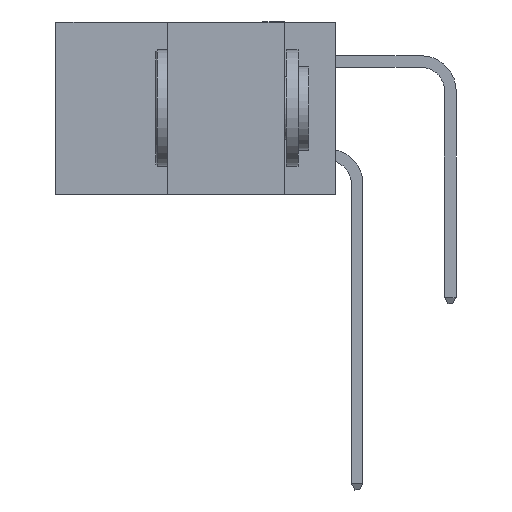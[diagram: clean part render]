
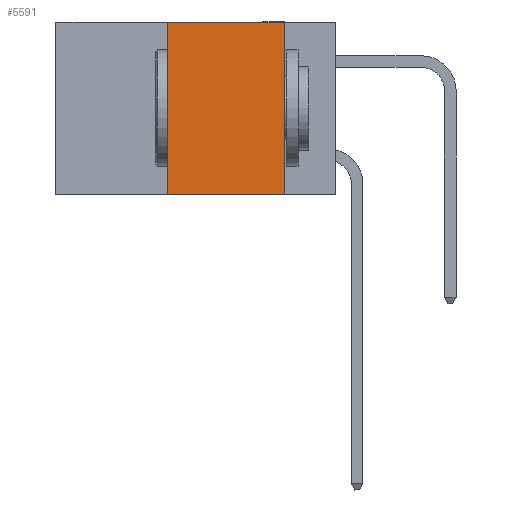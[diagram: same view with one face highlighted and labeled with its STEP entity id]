
A CAD part, left-side view. The second image highlights one B-rep face of the part: STEP entity #5591.
In plain terms, the highlighted planar face has unit normal (-1, 0, 0).
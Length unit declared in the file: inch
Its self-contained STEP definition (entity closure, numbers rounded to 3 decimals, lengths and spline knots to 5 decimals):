
#1608 = VECTOR ( 'NONE', #17284, 39.37008 ) ;
#1624 = LINE ( 'NONE', #6022, #5267 ) ;
#1703 = EDGE_LOOP ( 'NONE', ( #5693, #5803, #6019, #6111 ) ) ;
#1798 = CARTESIAN_POINT ( 'NONE',  ( 0., 0.6, 0. ) ) ;
#2608 = VECTOR ( 'NONE', #3394, 39.37008 ) ;
#2802 = VERTEX_POINT ( 'NONE', #12249 ) ;
#3334 = PLANE ( 'NONE',  #11237 ) ;
#3394 = DIRECTION ( 'NONE',  ( 0., -1., 0. ) ) ;
#5258 = VERTEX_POINT ( 'NONE', #11496 ) ;
#5267 = VECTOR ( 'NONE', #7521, 39.37008 ) ;
#5298 = CARTESIAN_POINT ( 'NONE',  ( 0., 0.11, 0. ) ) ;
#5416 = VECTOR ( 'NONE', #15651, 39.37008 ) ;
#5478 = CARTESIAN_POINT ( 'NONE',  ( 0., 0.6, -0.37 ) ) ;
#5591 = ADVANCED_FACE ( 'NONE', ( #16247 ), #3334, .F. ) ;
#5693 = ORIENTED_EDGE ( 'NONE', *, *, #8335, .F. ) ;
#5803 = ORIENTED_EDGE ( 'NONE', *, *, #16637, .F. ) ;
#6019 = ORIENTED_EDGE ( 'NONE', *, *, #7218, .F. ) ;
#6022 = CARTESIAN_POINT ( 'NONE',  ( 0., 0.36, 0. ) ) ;
#6111 = ORIENTED_EDGE ( 'NONE', *, *, #18169, .T. ) ;
#6213 = LINE ( 'NONE', #11580, #1608 ) ;
#6410 = DIRECTION ( 'NONE',  ( 0., 0., -1. ) ) ;
#6675 = LINE ( 'NONE', #1798, #2608 ) ;
#7218 = EDGE_CURVE ( 'NONE', #18068, #2802, #1624, .T. ) ;
#7521 = DIRECTION ( 'NONE',  ( 0., 0., 1. ) ) ;
#8335 = EDGE_CURVE ( 'NONE', #15106, #5258, #6213, .T. ) ;
#11237 = AXIS2_PLACEMENT_3D ( 'NONE', #13642, #15063, #6410 ) ;
#11496 = CARTESIAN_POINT ( 'NONE',  ( 0., 0.11, -0.37 ) ) ;
#11580 = CARTESIAN_POINT ( 'NONE',  ( 0., 0.11, 0. ) ) ;
#12249 = CARTESIAN_POINT ( 'NONE',  ( 0., 0.36, 0. ) ) ;
#12540 = CARTESIAN_POINT ( 'NONE',  ( 0., 0.36, -0.37 ) ) ;
#13642 = CARTESIAN_POINT ( 'NONE',  ( 0., 0.6, 0. ) ) ;
#15063 = DIRECTION ( 'NONE',  ( 1., 0., 0. ) ) ;
#15106 = VERTEX_POINT ( 'NONE', #5298 ) ;
#15651 = DIRECTION ( 'NONE',  ( 0., -1., 0. ) ) ;
#16247 = FACE_OUTER_BOUND ( 'NONE', #1703, .T. ) ;
#16535 = LINE ( 'NONE', #5478, #5416 ) ;
#16637 = EDGE_CURVE ( 'NONE', #2802, #15106, #6675, .T. ) ;
#17284 = DIRECTION ( 'NONE',  ( 0., 0., -1. ) ) ;
#18068 = VERTEX_POINT ( 'NONE', #12540 ) ;
#18169 = EDGE_CURVE ( 'NONE', #18068, #5258, #16535, .T. ) ;
